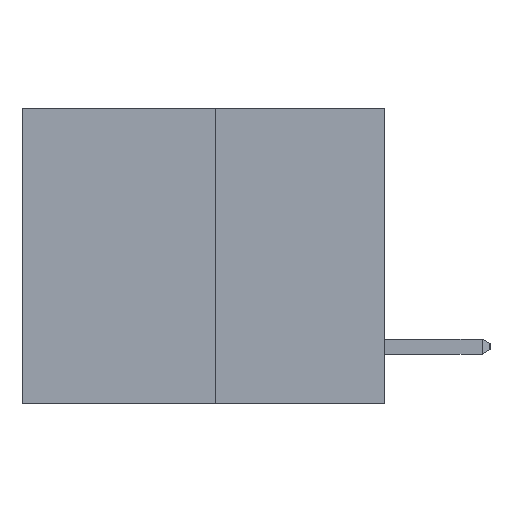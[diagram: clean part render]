
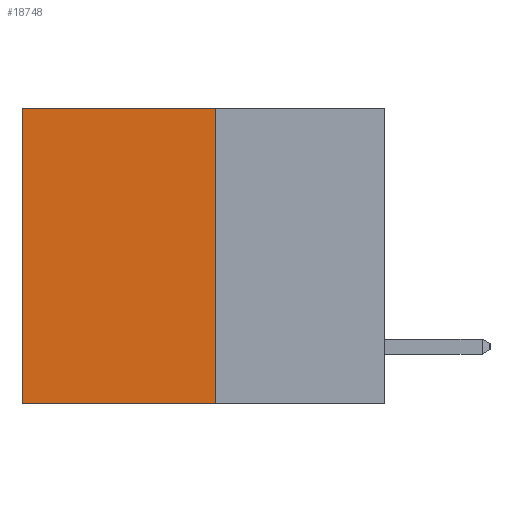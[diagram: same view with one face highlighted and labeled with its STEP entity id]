
A CAD part, left-side view. The second image highlights one B-rep face of the part: STEP entity #18748.
In plain terms, the highlighted planar face has unit normal (-1, 0, 0).
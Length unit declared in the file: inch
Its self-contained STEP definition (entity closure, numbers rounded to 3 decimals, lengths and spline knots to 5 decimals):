
#129 = VERTEX_POINT ( 'NONE', #13974 ) ;
#782 = DIRECTION ( 'NONE',  ( 0., 1., 0. ) ) ;
#1217 = DIRECTION ( 'NONE',  ( 0., 0., -1. ) ) ;
#2280 = VECTOR ( 'NONE', #25516, 39.37008 ) ;
#2818 = VERTEX_POINT ( 'NONE', #4149 ) ;
#3081 = CARTESIAN_POINT ( 'NONE',  ( 0.3165, 0.6, -0.49 ) ) ;
#3416 = CARTESIAN_POINT ( 'NONE',  ( 0.3165, 0.28, -0.49 ) ) ;
#3503 = PLANE ( 'NONE',  #25741 ) ;
#4149 = CARTESIAN_POINT ( 'NONE',  ( 0.3165, 0.6, 0. ) ) ;
#4291 = ORIENTED_EDGE ( 'NONE', *, *, #23196, .T. ) ;
#4340 = EDGE_CURVE ( 'NONE', #129, #22245, #21199, .T. ) ;
#5515 = DIRECTION ( 'NONE',  ( 1., 0., 0. ) ) ;
#7199 = DIRECTION ( 'NONE',  ( 0., 0., -1. ) ) ;
#7223 = VECTOR ( 'NONE', #7199, 39.37008 ) ;
#9772 = VECTOR ( 'NONE', #1217, 39.37008 ) ;
#10648 = EDGE_CURVE ( 'NONE', #21746, #2818, #12968, .T. ) ;
#12370 = CARTESIAN_POINT ( 'NONE',  ( 0.3165, 0.28, 0. ) ) ;
#12838 = CARTESIAN_POINT ( 'NONE',  ( 0.3165, 0.28, -0.49 ) ) ;
#12968 = LINE ( 'NONE', #23484, #2280 ) ;
#13216 = LINE ( 'NONE', #3081, #9772 ) ;
#13476 = EDGE_LOOP ( 'NONE', ( #4291, #17107, #25965, #23099 ) ) ;
#13537 = FACE_OUTER_BOUND ( 'NONE', #13476, .T. ) ;
#13974 = CARTESIAN_POINT ( 'NONE',  ( 0.3165, 0.28, -0.49 ) ) ;
#15767 = CARTESIAN_POINT ( 'NONE',  ( 0.3165, 0.6, -0.49 ) ) ;
#17107 = ORIENTED_EDGE ( 'NONE', *, *, #4340, .F. ) ;
#18365 = VECTOR ( 'NONE', #782, 39.37008 ) ;
#18748 = ADVANCED_FACE ( 'NONE', ( #13537 ), #3503, .F. ) ;
#19176 = LINE ( 'NONE', #19246, #7223 ) ;
#19246 = CARTESIAN_POINT ( 'NONE',  ( 0.3165, 0.28, -0.49 ) ) ;
#21199 = LINE ( 'NONE', #12838, #18365 ) ;
#21278 = DIRECTION ( 'NONE',  ( 0., 0., -1. ) ) ;
#21746 = VERTEX_POINT ( 'NONE', #12370 ) ;
#22245 = VERTEX_POINT ( 'NONE', #15767 ) ;
#23099 = ORIENTED_EDGE ( 'NONE', *, *, #10648, .T. ) ;
#23196 = EDGE_CURVE ( 'NONE', #2818, #22245, #13216, .T. ) ;
#23279 = EDGE_CURVE ( 'NONE', #21746, #129, #19176, .T. ) ;
#23484 = CARTESIAN_POINT ( 'NONE',  ( 0.3165, 0.28, 0. ) ) ;
#25516 = DIRECTION ( 'NONE',  ( 0., 1., 0. ) ) ;
#25741 = AXIS2_PLACEMENT_3D ( 'NONE', #3416, #5515, #21278 ) ;
#25965 = ORIENTED_EDGE ( 'NONE', *, *, #23279, .F. ) ;
